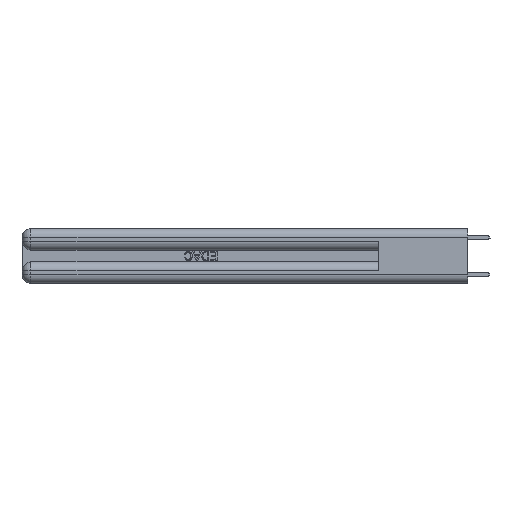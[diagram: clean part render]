
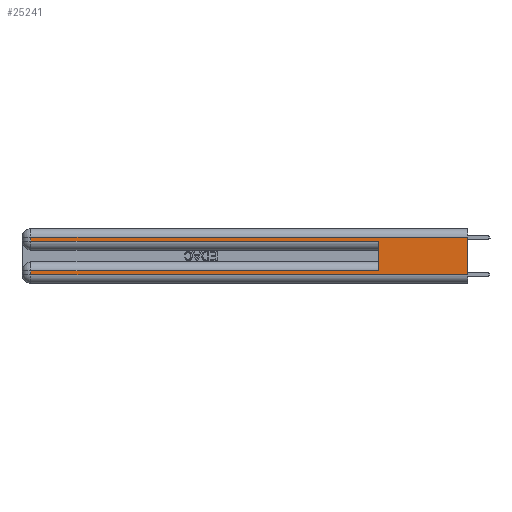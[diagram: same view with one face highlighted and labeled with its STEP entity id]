
A CAD part, left-side view. The second image highlights one B-rep face of the part: STEP entity #25241.
In plain terms, the highlighted planar face has unit normal (-1, 0, 0).
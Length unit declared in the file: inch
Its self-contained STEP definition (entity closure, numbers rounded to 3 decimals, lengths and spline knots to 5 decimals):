
#1478 = CARTESIAN_POINT ( 'NONE',  ( 0., 2.94, 0.31 ) ) ;
#1700 = EDGE_CURVE ( 'NONE', #21508, #13401, #6899, .T. ) ;
#2333 = VERTEX_POINT ( 'NONE', #32279 ) ;
#2571 = DIRECTION ( 'NONE',  ( 0., 0., 1. ) ) ;
#2726 = ORIENTED_EDGE ( 'NONE', *, *, #28102, .T. ) ;
#2759 = VECTOR ( 'NONE', #2571, 39.37008 ) ;
#3341 = ORIENTED_EDGE ( 'NONE', *, *, #30262, .F. ) ;
#3796 = CARTESIAN_POINT ( 'NONE',  ( 0., 0., 0.31 ) ) ;
#3879 = DIRECTION ( 'NONE',  ( 0., -1., 0. ) ) ;
#3999 = CARTESIAN_POINT ( 'NONE',  ( 0., 0., 0.285 ) ) ;
#4841 = LINE ( 'NONE', #7726, #2759 ) ;
#5587 = VECTOR ( 'NONE', #7525, 39.37008 ) ;
#6284 = VECTOR ( 'NONE', #29198, 39.37008 ) ;
#6486 = CARTESIAN_POINT ( 'NONE',  ( 0., 0.6, 0.085 ) ) ;
#6845 = EDGE_CURVE ( 'NONE', #2333, #21377, #27184, .T. ) ;
#6899 = LINE ( 'NONE', #3999, #11936 ) ;
#7525 = DIRECTION ( 'NONE',  ( 0., 0., -1. ) ) ;
#7609 = CARTESIAN_POINT ( 'NONE',  ( 0., 2.94, 0.37 ) ) ;
#7726 = CARTESIAN_POINT ( 'NONE',  ( 0., 0.6, 0.145 ) ) ;
#9638 = FACE_OUTER_BOUND ( 'NONE', #27023, .T. ) ;
#10789 = LINE ( 'NONE', #19943, #19651 ) ;
#11216 = VECTOR ( 'NONE', #21238, 39.37008 ) ;
#11428 = EDGE_CURVE ( 'NONE', #17876, #20138, #10789, .T. ) ;
#11936 = VECTOR ( 'NONE', #3879, 39.37008 ) ;
#13227 = PLANE ( 'NONE',  #25175 ) ;
#13401 = VERTEX_POINT ( 'NONE', #32571 ) ;
#13458 = CARTESIAN_POINT ( 'NONE',  ( 0., 0., 0.06 ) ) ;
#13572 = DIRECTION ( 'NONE',  ( 1., 0., 0. ) ) ;
#13751 = EDGE_CURVE ( 'NONE', #17876, #18198, #32862, .T. ) ;
#14194 = VERTEX_POINT ( 'NONE', #6486 ) ;
#14627 = ORIENTED_EDGE ( 'NONE', *, *, #13751, .F. ) ;
#14891 = DIRECTION ( 'NONE',  ( 0., 1., 0. ) ) ;
#16388 = EDGE_CURVE ( 'NONE', #14194, #2333, #18474, .T. ) ;
#17876 = VERTEX_POINT ( 'NONE', #3796 ) ;
#18198 = VERTEX_POINT ( 'NONE', #32488 ) ;
#18228 = ORIENTED_EDGE ( 'NONE', *, *, #11428, .T. ) ;
#18474 = LINE ( 'NONE', #18510, #6284 ) ;
#18510 = CARTESIAN_POINT ( 'NONE',  ( 0., 0., 0.085 ) ) ;
#18724 = CARTESIAN_POINT ( 'NONE',  ( 0., 0., 0.37 ) ) ;
#19121 = CARTESIAN_POINT ( 'NONE',  ( 0., 2.94, 0.285 ) ) ;
#19651 = VECTOR ( 'NONE', #14891, 39.37008 ) ;
#19676 = ORIENTED_EDGE ( 'NONE', *, *, #1700, .T. ) ;
#19943 = CARTESIAN_POINT ( 'NONE',  ( 0., 0., 0.31 ) ) ;
#20138 = VERTEX_POINT ( 'NONE', #1478 ) ;
#20565 = EDGE_CURVE ( 'NONE', #20138, #21508, #25360, .T. ) ;
#21238 = DIRECTION ( 'NONE',  ( 0., -1., 0. ) ) ;
#21377 = VERTEX_POINT ( 'NONE', #26525 ) ;
#21473 = DIRECTION ( 'NONE',  ( 0., 0., -1. ) ) ;
#21508 = VERTEX_POINT ( 'NONE', #19121 ) ;
#21751 = VECTOR ( 'NONE', #26890, 39.37008 ) ;
#23631 = CARTESIAN_POINT ( 'NONE',  ( 0., 2.94, 0.37 ) ) ;
#24972 = VECTOR ( 'NONE', #28838, 39.37008 ) ;
#25175 = AXIS2_PLACEMENT_3D ( 'NONE', #18724, #13572, #21473 ) ;
#25241 = ADVANCED_FACE ( 'NONE', ( #9638 ), #13227, .F. ) ;
#25360 = LINE ( 'NONE', #23631, #5587 ) ;
#25705 = CARTESIAN_POINT ( 'NONE',  ( 0., 0., 0.37 ) ) ;
#25821 = ORIENTED_EDGE ( 'NONE', *, *, #20565, .T. ) ;
#26525 = CARTESIAN_POINT ( 'NONE',  ( 0., 2.94, 0.06 ) ) ;
#26890 = DIRECTION ( 'NONE',  ( 0., 0., -1. ) ) ;
#27023 = EDGE_LOOP ( 'NONE', ( #14627, #18228, #25821, #19676, #3341, #28348, #32269, #2726 ) ) ;
#27184 = LINE ( 'NONE', #7609, #21751 ) ;
#28102 = EDGE_CURVE ( 'NONE', #21377, #18198, #31391, .T. ) ;
#28348 = ORIENTED_EDGE ( 'NONE', *, *, #16388, .T. ) ;
#28838 = DIRECTION ( 'NONE',  ( 0., 0., -1. ) ) ;
#29198 = DIRECTION ( 'NONE',  ( 0., 1., 0. ) ) ;
#30262 = EDGE_CURVE ( 'NONE', #14194, #13401, #4841, .T. ) ;
#31391 = LINE ( 'NONE', #13458, #11216 ) ;
#32269 = ORIENTED_EDGE ( 'NONE', *, *, #6845, .T. ) ;
#32279 = CARTESIAN_POINT ( 'NONE',  ( 0., 2.94, 0.085 ) ) ;
#32488 = CARTESIAN_POINT ( 'NONE',  ( 0., 0., 0.06 ) ) ;
#32571 = CARTESIAN_POINT ( 'NONE',  ( 0., 0.6, 0.285 ) ) ;
#32862 = LINE ( 'NONE', #25705, #24972 ) ;
